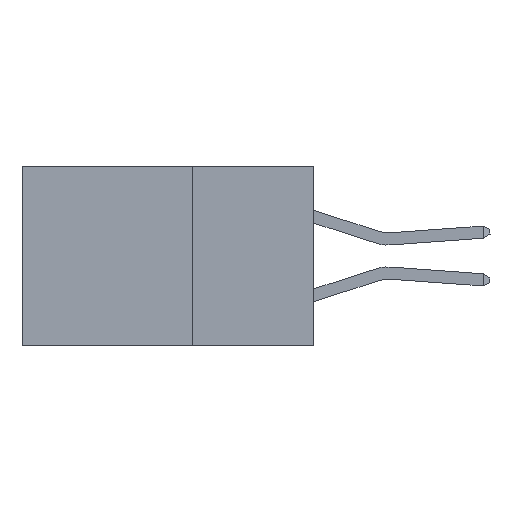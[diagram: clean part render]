
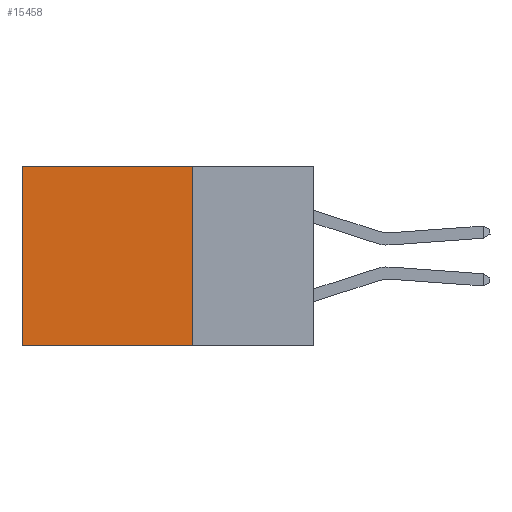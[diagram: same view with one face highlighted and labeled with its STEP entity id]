
A CAD part, left-side view. The second image highlights one B-rep face of the part: STEP entity #15458.
In plain terms, the highlighted planar face has unit normal (-1, 0, 0).
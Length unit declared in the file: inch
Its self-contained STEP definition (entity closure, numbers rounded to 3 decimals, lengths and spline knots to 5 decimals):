
#98 = VERTEX_POINT ( 'NONE', #10581 ) ;
#305 = CARTESIAN_POINT ( 'NONE',  ( 0.2875, 0.25, -0.37 ) ) ;
#606 = EDGE_CURVE ( 'NONE', #12364, #11716, #2170, .T. ) ;
#1692 = VECTOR ( 'NONE', #11333, 39.37008 ) ;
#1791 = DIRECTION ( 'NONE',  ( 1., 0., 0. ) ) ;
#2170 = LINE ( 'NONE', #10762, #1692 ) ;
#2282 = ORIENTED_EDGE ( 'NONE', *, *, #14564, .T. ) ;
#2899 = EDGE_CURVE ( 'NONE', #6051, #98, #7424, .T. ) ;
#2953 = AXIS2_PLACEMENT_3D ( 'NONE', #9244, #1791, #12243 ) ;
#3716 = ORIENTED_EDGE ( 'NONE', *, *, #8634, .F. ) ;
#4226 = CARTESIAN_POINT ( 'NONE',  ( 0.2875, 0.25, 0. ) ) ;
#4253 = EDGE_LOOP ( 'NONE', ( #2282, #6532, #3716, #10523 ) ) ;
#4299 = CARTESIAN_POINT ( 'NONE',  ( 0.2875, 0.25, 0. ) ) ;
#5322 = LINE ( 'NONE', #4299, #17739 ) ;
#5733 = DIRECTION ( 'NONE',  ( 0., 1., 0. ) ) ;
#6051 = VERTEX_POINT ( 'NONE', #305 ) ;
#6532 = ORIENTED_EDGE ( 'NONE', *, *, #2899, .F. ) ;
#7424 = LINE ( 'NONE', #8659, #10901 ) ;
#8596 = FACE_OUTER_BOUND ( 'NONE', #4253, .T. ) ;
#8628 = VECTOR ( 'NONE', #17613, 39.37008 ) ;
#8634 = EDGE_CURVE ( 'NONE', #12364, #6051, #5322, .T. ) ;
#8659 = CARTESIAN_POINT ( 'NONE',  ( 0.2875, 0.25, -0.37 ) ) ;
#9095 = LINE ( 'NONE', #16161, #8628 ) ;
#9244 = CARTESIAN_POINT ( 'NONE',  ( 0.2875, 0.25, 0. ) ) ;
#10523 = ORIENTED_EDGE ( 'NONE', *, *, #606, .T. ) ;
#10581 = CARTESIAN_POINT ( 'NONE',  ( 0.2875, 0.6, -0.37 ) ) ;
#10762 = CARTESIAN_POINT ( 'NONE',  ( 0.2875, 0.25, 0. ) ) ;
#10901 = VECTOR ( 'NONE', #5733, 39.37008 ) ;
#11333 = DIRECTION ( 'NONE',  ( 0., 1., 0. ) ) ;
#11716 = VERTEX_POINT ( 'NONE', #15943 ) ;
#12243 = DIRECTION ( 'NONE',  ( 0., 0., -1. ) ) ;
#12364 = VERTEX_POINT ( 'NONE', #4226 ) ;
#14564 = EDGE_CURVE ( 'NONE', #11716, #98, #9095, .T. ) ;
#15458 = ADVANCED_FACE ( 'NONE', ( #8596 ), #16730, .F. ) ;
#15943 = CARTESIAN_POINT ( 'NONE',  ( 0.2875, 0.6, 0. ) ) ;
#16161 = CARTESIAN_POINT ( 'NONE',  ( 0.2875, 0.6, 0. ) ) ;
#16261 = DIRECTION ( 'NONE',  ( 0., 0., -1. ) ) ;
#16730 = PLANE ( 'NONE',  #2953 ) ;
#17613 = DIRECTION ( 'NONE',  ( 0., 0., -1. ) ) ;
#17739 = VECTOR ( 'NONE', #16261, 39.37008 ) ;
